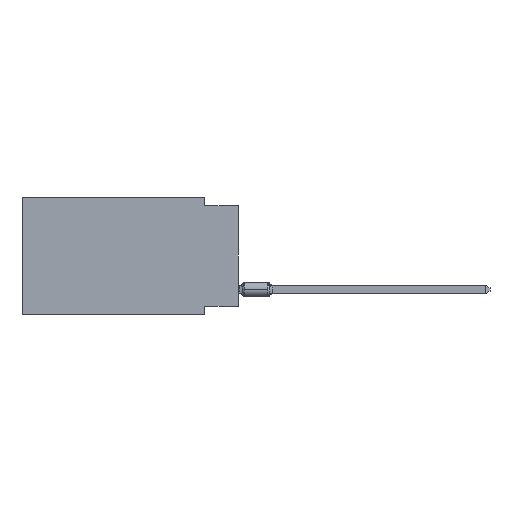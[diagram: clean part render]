
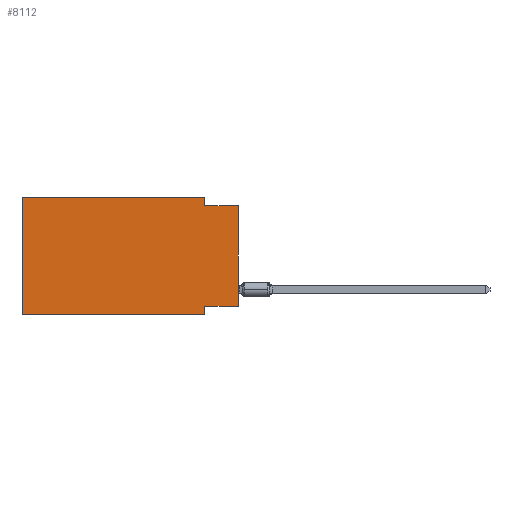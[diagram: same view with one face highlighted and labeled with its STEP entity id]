
A CAD part, left-side view. The second image highlights one B-rep face of the part: STEP entity #8112.
In plain terms, the highlighted planar face has unit normal (-1, 0, 0).
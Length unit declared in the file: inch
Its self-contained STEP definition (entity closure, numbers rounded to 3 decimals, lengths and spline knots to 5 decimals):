
#235 = ORIENTED_EDGE ( 'NONE', *, *, #413, .F. ) ;
#283 = CARTESIAN_POINT ( 'NONE',  ( 0., 0., -0.025 ) ) ;
#413 = EDGE_CURVE ( 'NONE', #3479, #3849, #576, .T. ) ;
#442 = LINE ( 'NONE', #14743, #12970 ) ;
#544 = VECTOR ( 'NONE', #6369, 39.37008 ) ;
#576 = LINE ( 'NONE', #8196, #11073 ) ;
#743 = LINE ( 'NONE', #9616, #15810 ) ;
#805 = CARTESIAN_POINT ( 'NONE',  ( 0., 0.1, -0.35 ) ) ;
#995 = ORIENTED_EDGE ( 'NONE', *, *, #11456, .F. ) ;
#1348 = DIRECTION ( 'NONE',  ( 0., 1., 0. ) ) ;
#2036 = ORIENTED_EDGE ( 'NONE', *, *, #5191, .F. ) ;
#2218 = ORIENTED_EDGE ( 'NONE', *, *, #4114, .F. ) ;
#2572 = ORIENTED_EDGE ( 'NONE', *, *, #3998, .F. ) ;
#3061 = VECTOR ( 'NONE', #11018, 39.37008 ) ;
#3194 = ORIENTED_EDGE ( 'NONE', *, *, #12683, .T. ) ;
#3199 = CARTESIAN_POINT ( 'NONE',  ( 0., 0.1, -0.35 ) ) ;
#3223 = EDGE_CURVE ( 'NONE', #15784, #10087, #16049, .T. ) ;
#3283 = DIRECTION ( 'NONE',  ( 0., 0., -1. ) ) ;
#3479 = VERTEX_POINT ( 'NONE', #11603 ) ;
#3849 = VERTEX_POINT ( 'NONE', #15267 ) ;
#3998 = EDGE_CURVE ( 'NONE', #16534, #14779, #14168, .T. ) ;
#4041 = LINE ( 'NONE', #6782, #16299 ) ;
#4114 = EDGE_CURVE ( 'NONE', #7162, #16534, #442, .T. ) ;
#4145 = DIRECTION ( 'NONE',  ( 0., -1., 0. ) ) ;
#4175 = DIRECTION ( 'NONE',  ( 1., 0., 0. ) ) ;
#4227 = LINE ( 'NONE', #9404, #8234 ) ;
#4796 = ORIENTED_EDGE ( 'NONE', *, *, #3223, .F. ) ;
#5191 = EDGE_CURVE ( 'NONE', #3849, #7162, #4227, .T. ) ;
#5501 = DIRECTION ( 'NONE',  ( 0., 0., -1. ) ) ;
#5743 = CARTESIAN_POINT ( 'NONE',  ( 0., 0.645, 0. ) ) ;
#6369 = DIRECTION ( 'NONE',  ( 0., 0., 1. ) ) ;
#6782 = CARTESIAN_POINT ( 'NONE',  ( 0., 0., -0.325 ) ) ;
#7162 = VERTEX_POINT ( 'NONE', #13824 ) ;
#7522 = CARTESIAN_POINT ( 'NONE',  ( 0., 0.1, -0.025 ) ) ;
#7685 = AXIS2_PLACEMENT_3D ( 'NONE', #5743, #4175, #5501 ) ;
#8112 = ADVANCED_FACE ( 'NONE', ( #14454 ), #8254, .F. ) ;
#8196 = CARTESIAN_POINT ( 'NONE',  ( 0., 0.645, 0. ) ) ;
#8234 = VECTOR ( 'NONE', #11906, 39.37008 ) ;
#8254 = PLANE ( 'NONE',  #7685 ) ;
#8738 = CARTESIAN_POINT ( 'NONE',  ( 0., 0., -0.325 ) ) ;
#9404 = CARTESIAN_POINT ( 'NONE',  ( 0., 0.645, 0. ) ) ;
#9616 = CARTESIAN_POINT ( 'NONE',  ( 0., 0.645, -0.35 ) ) ;
#10087 = VERTEX_POINT ( 'NONE', #3199 ) ;
#10120 = ORIENTED_EDGE ( 'NONE', *, *, #13811, .T. ) ;
#10568 = VECTOR ( 'NONE', #4145, 39.37008 ) ;
#11018 = DIRECTION ( 'NONE',  ( 0., 0., -1. ) ) ;
#11073 = VECTOR ( 'NONE', #13299, 39.37008 ) ;
#11225 = LINE ( 'NONE', #12816, #544 ) ;
#11456 = EDGE_CURVE ( 'NONE', #12170, #15784, #4041, .T. ) ;
#11603 = CARTESIAN_POINT ( 'NONE',  ( 0., 0.645, -0.35 ) ) ;
#11906 = DIRECTION ( 'NONE',  ( 0., -1., 0. ) ) ;
#12109 = EDGE_LOOP ( 'NONE', ( #3194, #2572, #2218, #2036, #235, #10120, #4796, #995 ) ) ;
#12170 = VERTEX_POINT ( 'NONE', #8738 ) ;
#12211 = DIRECTION ( 'NONE',  ( 0., -1., 0. ) ) ;
#12683 = EDGE_CURVE ( 'NONE', #12170, #14779, #11225, .T. ) ;
#12774 = CARTESIAN_POINT ( 'NONE',  ( 0., 0.1, -0.325 ) ) ;
#12816 = CARTESIAN_POINT ( 'NONE',  ( 0., 0., 0. ) ) ;
#12970 = VECTOR ( 'NONE', #3283, 39.37008 ) ;
#13299 = DIRECTION ( 'NONE',  ( 0., 0., 1. ) ) ;
#13650 = CARTESIAN_POINT ( 'NONE',  ( 0., 0., -0.025 ) ) ;
#13811 = EDGE_CURVE ( 'NONE', #3479, #10087, #743, .T. ) ;
#13824 = CARTESIAN_POINT ( 'NONE',  ( 0., 0.1, 0. ) ) ;
#14168 = LINE ( 'NONE', #283, #10568 ) ;
#14454 = FACE_OUTER_BOUND ( 'NONE', #12109, .T. ) ;
#14743 = CARTESIAN_POINT ( 'NONE',  ( 0., 0.1, 0. ) ) ;
#14779 = VERTEX_POINT ( 'NONE', #13650 ) ;
#15267 = CARTESIAN_POINT ( 'NONE',  ( 0., 0.645, 0. ) ) ;
#15784 = VERTEX_POINT ( 'NONE', #12774 ) ;
#15810 = VECTOR ( 'NONE', #12211, 39.37008 ) ;
#16049 = LINE ( 'NONE', #805, #3061 ) ;
#16299 = VECTOR ( 'NONE', #1348, 39.37008 ) ;
#16534 = VERTEX_POINT ( 'NONE', #7522 ) ;
